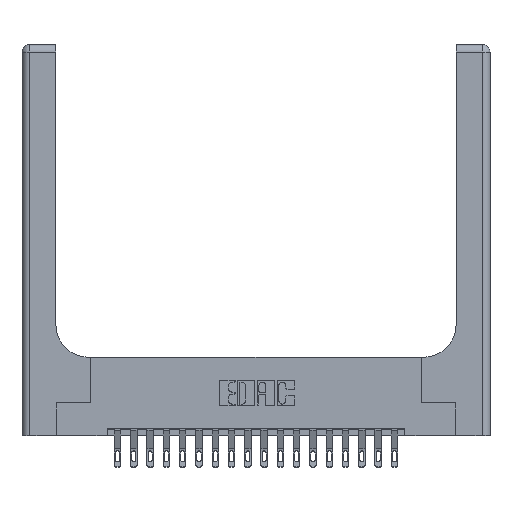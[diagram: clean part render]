
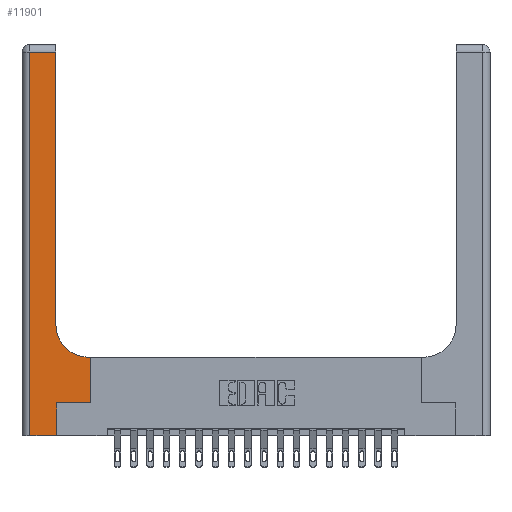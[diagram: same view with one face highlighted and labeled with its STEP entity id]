
A CAD part, top view. The second image highlights one B-rep face of the part: STEP entity #11901.
In plain terms, the highlighted planar face has unit normal (0, 0, 1).
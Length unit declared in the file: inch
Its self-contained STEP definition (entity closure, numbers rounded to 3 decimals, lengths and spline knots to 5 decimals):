
#251 = DIRECTION ( 'NONE',  ( 1., 0., 0. ) ) ;
#1136 = CARTESIAN_POINT ( 'NONE',  ( 0.26, 2.94, 0.37 ) ) ;
#1174 = DIRECTION ( 'NONE',  ( -1., 0., 0. ) ) ;
#1527 = CARTESIAN_POINT ( 'NONE',  ( 0.26, 0.6, 0.37 ) ) ;
#1616 = VERTEX_POINT ( 'NONE', #16221 ) ;
#1641 = VERTEX_POINT ( 'NONE', #1782 ) ;
#1737 = CARTESIAN_POINT ( 'NONE',  ( 0.06, 2.94, 0.37 ) ) ;
#1782 = CARTESIAN_POINT ( 'NONE',  ( 0.265, 0., 0.37 ) ) ;
#2466 = VERTEX_POINT ( 'NONE', #1136 ) ;
#3017 = CARTESIAN_POINT ( 'NONE',  ( 0.528, 0.25, 0.37 ) ) ;
#3320 = VERTEX_POINT ( 'NONE', #1737 ) ;
#3600 = DIRECTION ( 'NONE',  ( 0., -1., 0. ) ) ;
#3741 = VERTEX_POINT ( 'NONE', #5098 ) ;
#3755 = DIRECTION ( 'NONE',  ( 1., 0., 0. ) ) ;
#4782 = ORIENTED_EDGE ( 'NONE', *, *, #17961, .T. ) ;
#5098 = CARTESIAN_POINT ( 'NONE',  ( 0.265, 0.25, 0.37 ) ) ;
#5327 = DIRECTION ( 'NONE',  ( 0., 1., 0. ) ) ;
#5392 = EDGE_CURVE ( 'NONE', #3320, #12814, #18276, .T. ) ;
#5690 = AXIS2_PLACEMENT_3D ( 'NONE', #9843, #14750, #251 ) ;
#6027 = EDGE_CURVE ( 'NONE', #3741, #7446, #19102, .T. ) ;
#6149 = DIRECTION ( 'NONE',  ( 0., 1., 0. ) ) ;
#6439 = LINE ( 'NONE', #1527, #9306 ) ;
#6746 = DIRECTION ( 'NONE',  ( -1., 0., 0. ) ) ;
#7007 = VECTOR ( 'NONE', #12734, 39.37008 ) ;
#7446 = VERTEX_POINT ( 'NONE', #8973 ) ;
#7616 = CARTESIAN_POINT ( 'NONE',  ( 0.265, 0., 0.37 ) ) ;
#7635 = LINE ( 'NONE', #3017, #8116 ) ;
#7899 = VECTOR ( 'NONE', #6746, 39.37008 ) ;
#7914 = DIRECTION ( 'NONE',  ( -1., 0., 0. ) ) ;
#8116 = VECTOR ( 'NONE', #19040, 39.37008 ) ;
#8330 = EDGE_CURVE ( 'NONE', #1616, #12783, #14833, .T. ) ;
#8759 = EDGE_CURVE ( 'NONE', #12814, #1641, #10552, .T. ) ;
#8832 = CARTESIAN_POINT ( 'NONE',  ( 0., 0., 0.37 ) ) ;
#8838 = DIRECTION ( 'NONE',  ( 0., 0., -1. ) ) ;
#8973 = CARTESIAN_POINT ( 'NONE',  ( 0.528, 0.25, 0.37 ) ) ;
#9059 = ORIENTED_EDGE ( 'NONE', *, *, #10846, .T. ) ;
#9160 = FACE_OUTER_BOUND ( 'NONE', #18993, .T. ) ;
#9306 = VECTOR ( 'NONE', #7914, 39.37008 ) ;
#9817 = LINE ( 'NONE', #16787, #7899 ) ;
#9843 = CARTESIAN_POINT ( 'NONE',  ( 0.51, 0.85, 0.37 ) ) ;
#10465 = EDGE_CURVE ( 'NONE', #7446, #14030, #7635, .T. ) ;
#10478 = VECTOR ( 'NONE', #3755, 39.37008 ) ;
#10552 = LINE ( 'NONE', #8832, #10478 ) ;
#10846 = EDGE_CURVE ( 'NONE', #12783, #2466, #18513, .T. ) ;
#11290 = ORIENTED_EDGE ( 'NONE', *, *, #8759, .T. ) ;
#11573 = AXIS2_PLACEMENT_3D ( 'NONE', #15685, #8838, #1174 ) ;
#11901 = ADVANCED_FACE ( 'NONE', ( #9160 ), #17064, .F. ) ;
#12355 = ORIENTED_EDGE ( 'NONE', *, *, #16761, .T. ) ;
#12587 = VECTOR ( 'NONE', #5327, 39.37008 ) ;
#12626 = CARTESIAN_POINT ( 'NONE',  ( 0.06, 0., 0.37 ) ) ;
#12734 = DIRECTION ( 'NONE',  ( 1., 0., 0. ) ) ;
#12783 = VERTEX_POINT ( 'NONE', #19005 ) ;
#12814 = VERTEX_POINT ( 'NONE', #12626 ) ;
#13480 = CARTESIAN_POINT ( 'NONE',  ( 0.06, 3., 0.37 ) ) ;
#13554 = ORIENTED_EDGE ( 'NONE', *, *, #10465, .T. ) ;
#13631 = EDGE_CURVE ( 'NONE', #1641, #3741, #20808, .T. ) ;
#13885 = ORIENTED_EDGE ( 'NONE', *, *, #6027, .T. ) ;
#14030 = VERTEX_POINT ( 'NONE', #17101 ) ;
#14307 = CARTESIAN_POINT ( 'NONE',  ( 0.265, 0.25, 0.37 ) ) ;
#14632 = VECTOR ( 'NONE', #6149, 39.37008 ) ;
#14750 = DIRECTION ( 'NONE',  ( 0., 0., -1. ) ) ;
#14833 = CIRCLE ( 'NONE', #5690, 0.25 ) ;
#15554 = VECTOR ( 'NONE', #3600, 39.37008 ) ;
#15587 = ORIENTED_EDGE ( 'NONE', *, *, #8330, .T. ) ;
#15685 = CARTESIAN_POINT ( 'NONE',  ( 0., 3., 0.37 ) ) ;
#16221 = CARTESIAN_POINT ( 'NONE',  ( 0.51, 0.6, 0.37 ) ) ;
#16761 = EDGE_CURVE ( 'NONE', #2466, #3320, #9817, .T. ) ;
#16787 = CARTESIAN_POINT ( 'NONE',  ( 0., 2.94, 0.37 ) ) ;
#17064 = PLANE ( 'NONE',  #11573 ) ;
#17101 = CARTESIAN_POINT ( 'NONE',  ( 0.528, 0.6, 0.37 ) ) ;
#17961 = EDGE_CURVE ( 'NONE', #14030, #1616, #6439, .T. ) ;
#18276 = LINE ( 'NONE', #13480, #15554 ) ;
#18513 = LINE ( 'NONE', #20183, #12587 ) ;
#18801 = ORIENTED_EDGE ( 'NONE', *, *, #13631, .T. ) ;
#18993 = EDGE_LOOP ( 'NONE', ( #9059, #12355, #19298, #11290, #18801, #13885, #13554, #4782, #15587 ) ) ;
#19005 = CARTESIAN_POINT ( 'NONE',  ( 0.26, 0.85, 0.37 ) ) ;
#19040 = DIRECTION ( 'NONE',  ( 0., 1., 0. ) ) ;
#19102 = LINE ( 'NONE', #14307, #7007 ) ;
#19298 = ORIENTED_EDGE ( 'NONE', *, *, #5392, .T. ) ;
#20183 = CARTESIAN_POINT ( 'NONE',  ( 0.26, 3., 0.37 ) ) ;
#20808 = LINE ( 'NONE', #7616, #14632 ) ;
